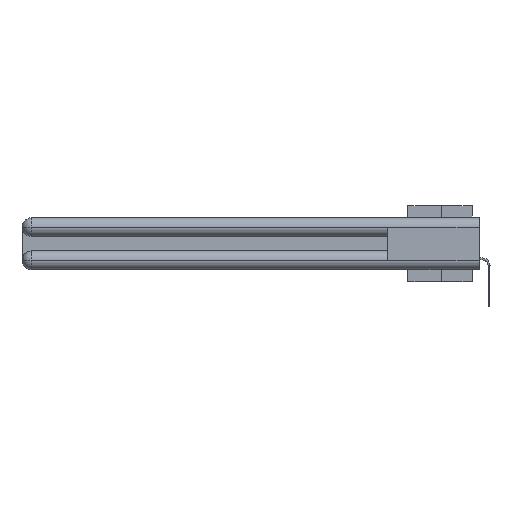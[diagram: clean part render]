
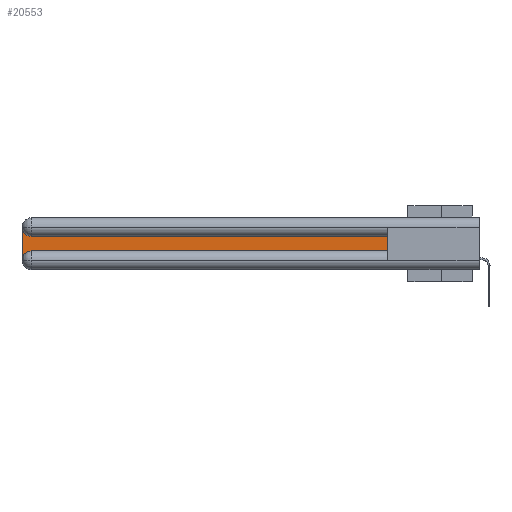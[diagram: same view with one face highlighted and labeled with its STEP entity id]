
A CAD part, left-side view. The second image highlights one B-rep face of the part: STEP entity #20553.
In plain terms, the highlighted planar face has unit normal (-1, 0, 0).
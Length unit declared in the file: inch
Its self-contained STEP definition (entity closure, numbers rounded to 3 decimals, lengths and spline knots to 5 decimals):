
#1291 = VERTEX_POINT ( 'NONE', #31999 ) ;
#1492 = EDGE_CURVE ( 'NONE', #37305, #28443, #33939, .T. ) ;
#1559 = DIRECTION ( 'NONE',  ( 0., -1., 0. ) ) ;
#4162 = VERTEX_POINT ( 'NONE', #18861 ) ;
#4362 = CARTESIAN_POINT ( 'NONE',  ( 0.075, 0.6, -0.1225 ) ) ;
#4580 = EDGE_CURVE ( 'NONE', #1291, #23669, #21195, .T. ) ;
#5201 = VECTOR ( 'NONE', #1559, 39.37008 ) ;
#5723 = CARTESIAN_POINT ( 'NONE',  ( 0.075, 2.94, -0.2175 ) ) ;
#5785 = CARTESIAN_POINT ( 'NONE',  ( 0.075, 3., -0.1225 ) ) ;
#6225 = AXIS2_PLACEMENT_3D ( 'NONE', #38490, #11464, #11655 ) ;
#6542 = CARTESIAN_POINT ( 'NONE',  ( 0.075, 3., -0.2775 ) ) ;
#6891 = CARTESIAN_POINT ( 'NONE',  ( 0.075, 0.6, -0.2175 ) ) ;
#7343 = ORIENTED_EDGE ( 'NONE', *, *, #12125, .T. ) ;
#9531 = VECTOR ( 'NONE', #31415, 39.37008 ) ;
#11439 = EDGE_CURVE ( 'NONE', #22499, #1291, #30616, .T. ) ;
#11464 = DIRECTION ( 'NONE',  ( 1., 0., 0. ) ) ;
#11655 = DIRECTION ( 'NONE',  ( 0., 0., -1. ) ) ;
#11856 = DIRECTION ( 'NONE',  ( 0., 0., -1. ) ) ;
#12125 = EDGE_CURVE ( 'NONE', #23669, #37305, #32523, .T. ) ;
#16436 = VECTOR ( 'NONE', #30336, 39.37008 ) ;
#16591 = AXIS2_PLACEMENT_3D ( 'NONE', #5785, #29496, #11856 ) ;
#18861 = CARTESIAN_POINT ( 'NONE',  ( 0.075, 0.6, -0.1225 ) ) ;
#19297 = EDGE_LOOP ( 'NONE', ( #29977, #30052, #28175, #7343, #24839, #37846 ) ) ;
#19620 = CARTESIAN_POINT ( 'NONE',  ( 0.075, 0.6, -0.2175 ) ) ;
#19863 = LINE ( 'NONE', #4362, #9531 ) ;
#20553 = ADVANCED_FACE ( 'NONE', ( #32637 ), #32448, .F. ) ;
#21195 = LINE ( 'NONE', #33517, #22939 ) ;
#21412 = DIRECTION ( 'NONE',  ( 1., 0., 0. ) ) ;
#21545 = CARTESIAN_POINT ( 'NONE',  ( 0.075, 0.6, -0.2175 ) ) ;
#22499 = VERTEX_POINT ( 'NONE', #31006 ) ;
#22939 = VECTOR ( 'NONE', #24715, 39.37008 ) ;
#23669 = VERTEX_POINT ( 'NONE', #6542 ) ;
#24352 = CARTESIAN_POINT ( 'NONE',  ( 0.075, 2.94, -0.0625 ) ) ;
#24715 = DIRECTION ( 'NONE',  ( 0., 0., -1. ) ) ;
#24839 = ORIENTED_EDGE ( 'NONE', *, *, #1492, .T. ) ;
#25616 = AXIS2_PLACEMENT_3D ( 'NONE', #24352, #21412, #33544 ) ;
#26204 = EDGE_CURVE ( 'NONE', #4162, #22499, #19863, .T. ) ;
#28175 = ORIENTED_EDGE ( 'NONE', *, *, #4580, .T. ) ;
#28443 = VERTEX_POINT ( 'NONE', #19620 ) ;
#29496 = DIRECTION ( 'NONE',  ( 1., 0., 0. ) ) ;
#29977 = ORIENTED_EDGE ( 'NONE', *, *, #26204, .T. ) ;
#30052 = ORIENTED_EDGE ( 'NONE', *, *, #11439, .T. ) ;
#30138 = LINE ( 'NONE', #21545, #16436 ) ;
#30336 = DIRECTION ( 'NONE',  ( 0., 0., 1. ) ) ;
#30616 = CIRCLE ( 'NONE', #25616, 0.06 ) ;
#31006 = CARTESIAN_POINT ( 'NONE',  ( 0.075, 2.94, -0.1225 ) ) ;
#31415 = DIRECTION ( 'NONE',  ( 0., 1., 0. ) ) ;
#31999 = CARTESIAN_POINT ( 'NONE',  ( 0.075, 3., -0.0625 ) ) ;
#32448 = PLANE ( 'NONE',  #16591 ) ;
#32523 = CIRCLE ( 'NONE', #6225, 0.06 ) ;
#32637 = FACE_OUTER_BOUND ( 'NONE', #19297, .T. ) ;
#33517 = CARTESIAN_POINT ( 'NONE',  ( 0.075, 3., -0.2175 ) ) ;
#33544 = DIRECTION ( 'NONE',  ( 0., 0., -1. ) ) ;
#33939 = LINE ( 'NONE', #6891, #5201 ) ;
#34222 = EDGE_CURVE ( 'NONE', #28443, #4162, #30138, .T. ) ;
#37305 = VERTEX_POINT ( 'NONE', #5723 ) ;
#37846 = ORIENTED_EDGE ( 'NONE', *, *, #34222, .T. ) ;
#38490 = CARTESIAN_POINT ( 'NONE',  ( 0.075, 2.94, -0.2775 ) ) ;
